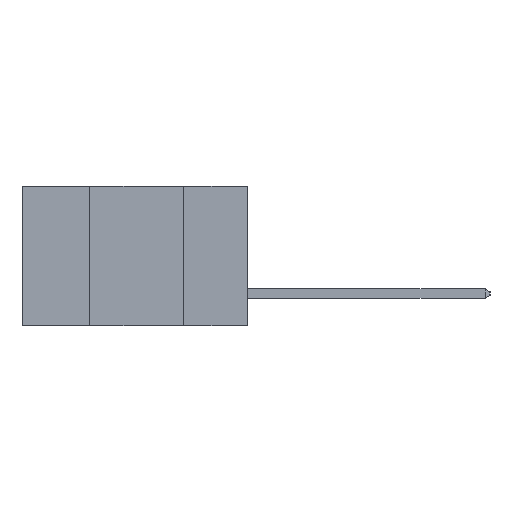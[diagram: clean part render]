
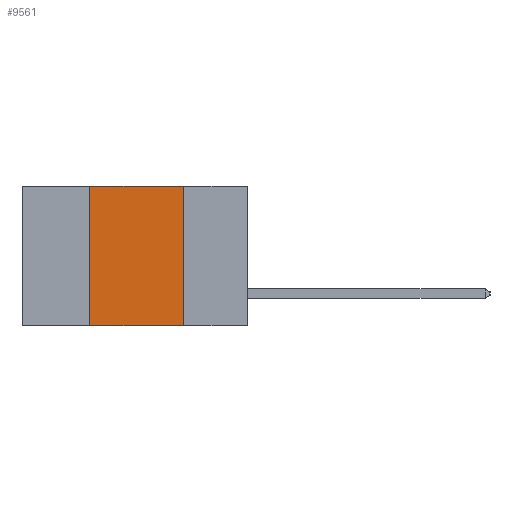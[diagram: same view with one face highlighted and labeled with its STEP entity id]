
A CAD part, left-side view. The second image highlights one B-rep face of the part: STEP entity #9561.
In plain terms, the highlighted planar face has unit normal (-1, 0, 0).
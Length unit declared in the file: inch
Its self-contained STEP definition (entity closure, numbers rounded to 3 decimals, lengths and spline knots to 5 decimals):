
#123 = VECTOR ( 'NONE', #8410, 39.37008 ) ;
#912 = FACE_OUTER_BOUND ( 'NONE', #7425, .T. ) ;
#1141 = VERTEX_POINT ( 'NONE', #7272 ) ;
#1418 = ORIENTED_EDGE ( 'NONE', *, *, #3899, .F. ) ;
#2149 = CARTESIAN_POINT ( 'NONE',  ( 0., 0.6, 0. ) ) ;
#2155 = EDGE_CURVE ( 'NONE', #12739, #10192, #5775, .T. ) ;
#3197 = ORIENTED_EDGE ( 'NONE', *, *, #14698, .F. ) ;
#3636 = CARTESIAN_POINT ( 'NONE',  ( 0., 0.42, -0.37 ) ) ;
#3899 = EDGE_CURVE ( 'NONE', #4571, #1141, #6900, .T. ) ;
#4235 = PLANE ( 'NONE',  #11715 ) ;
#4571 = VERTEX_POINT ( 'NONE', #15221 ) ;
#5063 = ORIENTED_EDGE ( 'NONE', *, *, #7264, .T. ) ;
#5399 = CARTESIAN_POINT ( 'NONE',  ( 0., 0.42, 0. ) ) ;
#5569 = DIRECTION ( 'NONE',  ( 1., 0., 0. ) ) ;
#5775 = LINE ( 'NONE', #12642, #11640 ) ;
#6900 = LINE ( 'NONE', #10754, #123 ) ;
#7244 = LINE ( 'NONE', #2149, #13773 ) ;
#7264 = EDGE_CURVE ( 'NONE', #12739, #1141, #10908, .T. ) ;
#7272 = CARTESIAN_POINT ( 'NONE',  ( 0., 0.17, -0.37 ) ) ;
#7425 = EDGE_LOOP ( 'NONE', ( #1418, #3197, #12211, #5063 ) ) ;
#7569 = DIRECTION ( 'NONE',  ( 0., -1., 0. ) ) ;
#8410 = DIRECTION ( 'NONE',  ( 0., 0., -1. ) ) ;
#9561 = ADVANCED_FACE ( 'NONE', ( #912 ), #4235, .F. ) ;
#10192 = VERTEX_POINT ( 'NONE', #5399 ) ;
#10632 = DIRECTION ( 'NONE',  ( 0., 0., 1. ) ) ;
#10754 = CARTESIAN_POINT ( 'NONE',  ( 0., 0.17, 0. ) ) ;
#10908 = LINE ( 'NONE', #12614, #13712 ) ;
#10984 = DIRECTION ( 'NONE',  ( 0., -1., 0. ) ) ;
#11640 = VECTOR ( 'NONE', #10632, 39.37008 ) ;
#11715 = AXIS2_PLACEMENT_3D ( 'NONE', #12997, #5569, #14172 ) ;
#12211 = ORIENTED_EDGE ( 'NONE', *, *, #2155, .F. ) ;
#12614 = CARTESIAN_POINT ( 'NONE',  ( 0., 0.6, -0.37 ) ) ;
#12642 = CARTESIAN_POINT ( 'NONE',  ( 0., 0.42, 0. ) ) ;
#12739 = VERTEX_POINT ( 'NONE', #3636 ) ;
#12997 = CARTESIAN_POINT ( 'NONE',  ( 0., 0.6, 0. ) ) ;
#13712 = VECTOR ( 'NONE', #7569, 39.37008 ) ;
#13773 = VECTOR ( 'NONE', #10984, 39.37008 ) ;
#14172 = DIRECTION ( 'NONE',  ( 0., 0., -1. ) ) ;
#14698 = EDGE_CURVE ( 'NONE', #10192, #4571, #7244, .T. ) ;
#15221 = CARTESIAN_POINT ( 'NONE',  ( 0., 0.17, 0. ) ) ;
